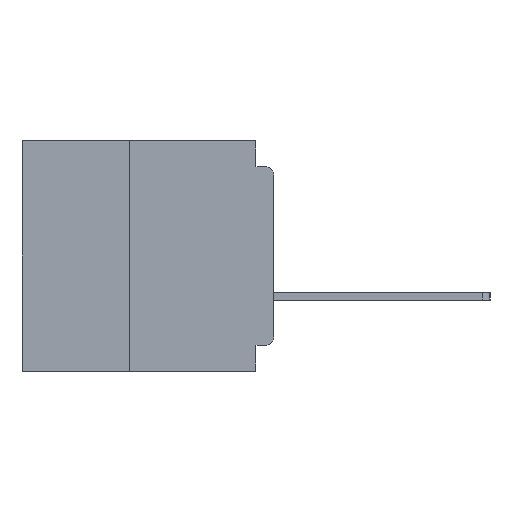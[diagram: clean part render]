
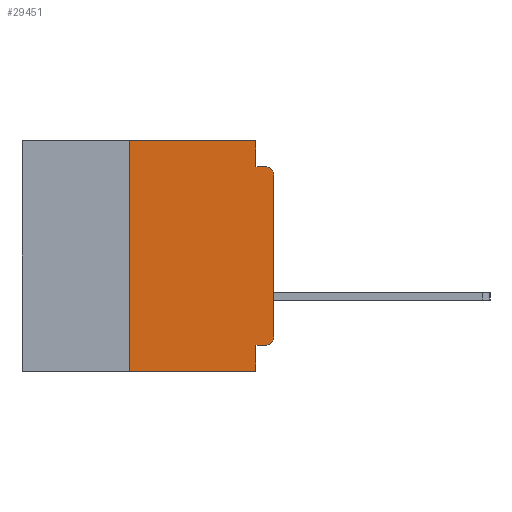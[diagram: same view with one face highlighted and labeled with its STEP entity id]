
A CAD part, left-side view. The second image highlights one B-rep face of the part: STEP entity #29451.
In plain terms, the highlighted planar face has unit normal (-1, 0, 0).
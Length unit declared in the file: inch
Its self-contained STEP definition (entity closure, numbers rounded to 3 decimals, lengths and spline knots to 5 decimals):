
#297 = VECTOR ( 'NONE', #43641, 39.37008 ) ;
#363 = DIRECTION ( 'NONE',  ( -1., 0., 0. ) ) ;
#499 = VERTEX_POINT ( 'NONE', #58375 ) ;
#901 = DIRECTION ( 'NONE',  ( 0., 0., -1. ) ) ;
#1110 = CARTESIAN_POINT ( 'NONE',  ( 0., 0.031, -0.4 ) ) ;
#2289 = CARTESIAN_POINT ( 'NONE',  ( 0., 0.031, -0.355 ) ) ;
#3205 = VERTEX_POINT ( 'NONE', #30571 ) ;
#4628 = EDGE_CURVE ( 'NONE', #499, #45607, #49005, .T. ) ;
#5086 = VECTOR ( 'NONE', #58828, 39.37008 ) ;
#6500 = EDGE_CURVE ( 'NONE', #499, #8777, #32813, .T. ) ;
#8254 = FACE_OUTER_BOUND ( 'NONE', #55263, .T. ) ;
#8302 = CARTESIAN_POINT ( 'NONE',  ( 0., 0., -0.34 ) ) ;
#8472 = CARTESIAN_POINT ( 'NONE',  ( 0., 0.031, -0.4 ) ) ;
#8777 = VERTEX_POINT ( 'NONE', #2289 ) ;
#8823 = VECTOR ( 'NONE', #19316, 39.37008 ) ;
#9510 = DIRECTION ( 'NONE',  ( 0., -1., 0. ) ) ;
#9801 = CARTESIAN_POINT ( 'NONE',  ( 0., 0., -0.045 ) ) ;
#10538 = ORIENTED_EDGE ( 'NONE', *, *, #6500, .F. ) ;
#11288 = ORIENTED_EDGE ( 'NONE', *, *, #31614, .T. ) ;
#12706 = ORIENTED_EDGE ( 'NONE', *, *, #37707, .F. ) ;
#13211 = VERTEX_POINT ( 'NONE', #19396 ) ;
#13712 = AXIS2_PLACEMENT_3D ( 'NONE', #56917, #27549, #61792 ) ;
#14845 = DIRECTION ( 'NONE',  ( 0., -1., 0. ) ) ;
#15233 = LINE ( 'NONE', #38761, #297 ) ;
#15885 = CARTESIAN_POINT ( 'NONE',  ( 0., 0.25, -0.4 ) ) ;
#19316 = DIRECTION ( 'NONE',  ( 0., 0., 1. ) ) ;
#19396 = CARTESIAN_POINT ( 'NONE',  ( 0., 0., -0.06 ) ) ;
#20513 = EDGE_CURVE ( 'NONE', #48472, #58981, #15233, .T. ) ;
#20899 = DIRECTION ( 'NONE',  ( 0., 0., 1. ) ) ;
#21132 = VECTOR ( 'NONE', #14845, 39.37008 ) ;
#23378 = CARTESIAN_POINT ( 'NONE',  ( 0., 0.031, 0. ) ) ;
#25372 = LINE ( 'NONE', #15885, #49978 ) ;
#26031 = VERTEX_POINT ( 'NONE', #8472 ) ;
#27549 = DIRECTION ( 'NONE',  ( -1., 0., 0. ) ) ;
#29451 = ADVANCED_FACE ( 'NONE', ( #8254 ), #57670, .F. ) ;
#29484 = CARTESIAN_POINT ( 'NONE',  ( 0., 0.437, -0.4 ) ) ;
#30360 = CARTESIAN_POINT ( 'NONE',  ( 0., 0.015, -0.34 ) ) ;
#30506 = ORIENTED_EDGE ( 'NONE', *, *, #43834, .T. ) ;
#30571 = CARTESIAN_POINT ( 'NONE',  ( 0., 0.25, 0. ) ) ;
#31138 = EDGE_CURVE ( 'NONE', #45115, #3205, #25372, .T. ) ;
#31614 = EDGE_CURVE ( 'NONE', #45607, #13211, #61322, .T. ) ;
#32395 = CARTESIAN_POINT ( 'NONE',  ( 0., 0.031, -0.045 ) ) ;
#32813 = LINE ( 'NONE', #50695, #58826 ) ;
#33079 = CARTESIAN_POINT ( 'NONE',  ( 0., 0.437, 0. ) ) ;
#33307 = DIRECTION ( 'NONE',  ( 0., 0., -1. ) ) ;
#34844 = LINE ( 'NONE', #29484, #5086 ) ;
#35324 = DIRECTION ( 'NONE',  ( 0., 0., -1. ) ) ;
#37707 = EDGE_CURVE ( 'NONE', #58981, #37766, #60367, .T. ) ;
#37766 = VERTEX_POINT ( 'NONE', #44688 ) ;
#38193 = ORIENTED_EDGE ( 'NONE', *, *, #51375, .T. ) ;
#38761 = CARTESIAN_POINT ( 'NONE',  ( 0., 0.031, 0. ) ) ;
#39537 = ORIENTED_EDGE ( 'NONE', *, *, #31138, .F. ) ;
#43641 = DIRECTION ( 'NONE',  ( 0., 0., -1. ) ) ;
#43834 = EDGE_CURVE ( 'NONE', #13211, #37766, #56960, .T. ) ;
#44688 = CARTESIAN_POINT ( 'NONE',  ( 0., 0.015, -0.045 ) ) ;
#45115 = VERTEX_POINT ( 'NONE', #58703 ) ;
#45207 = VECTOR ( 'NONE', #9510, 39.37008 ) ;
#45607 = VERTEX_POINT ( 'NONE', #8302 ) ;
#46761 = LINE ( 'NONE', #49159, #45207 ) ;
#47475 = AXIS2_PLACEMENT_3D ( 'NONE', #30360, #363, #35324 ) ;
#48472 = VERTEX_POINT ( 'NONE', #23378 ) ;
#48823 = ORIENTED_EDGE ( 'NONE', *, *, #4628, .T. ) ;
#48880 = LINE ( 'NONE', #1110, #61831 ) ;
#49005 = CIRCLE ( 'NONE', #47475, 0.015 ) ;
#49159 = CARTESIAN_POINT ( 'NONE',  ( 0., 0.437, 0. ) ) ;
#49428 = EDGE_CURVE ( 'NONE', #8777, #26031, #48880, .T. ) ;
#49978 = VECTOR ( 'NONE', #20899, 39.37008 ) ;
#50152 = AXIS2_PLACEMENT_3D ( 'NONE', #33079, #62545, #33307 ) ;
#50695 = CARTESIAN_POINT ( 'NONE',  ( 0., 0., -0.355 ) ) ;
#51375 = EDGE_CURVE ( 'NONE', #45115, #26031, #34844, .T. ) ;
#53790 = CARTESIAN_POINT ( 'NONE',  ( 0., 0., 0. ) ) ;
#54299 = EDGE_CURVE ( 'NONE', #3205, #48472, #46761, .T. ) ;
#55263 = EDGE_LOOP ( 'NONE', ( #11288, #30506, #12706, #61041, #61130, #39537, #38193, #57351, #10538, #48823 ) ) ;
#55634 = DIRECTION ( 'NONE',  ( 0., 1., 0. ) ) ;
#56917 = CARTESIAN_POINT ( 'NONE',  ( 0., 0.015, -0.06 ) ) ;
#56960 = CIRCLE ( 'NONE', #13712, 0.015 ) ;
#57351 = ORIENTED_EDGE ( 'NONE', *, *, #49428, .F. ) ;
#57670 = PLANE ( 'NONE',  #50152 ) ;
#58375 = CARTESIAN_POINT ( 'NONE',  ( 0., 0.015, -0.355 ) ) ;
#58703 = CARTESIAN_POINT ( 'NONE',  ( 0., 0.25, -0.4 ) ) ;
#58826 = VECTOR ( 'NONE', #55634, 39.37008 ) ;
#58828 = DIRECTION ( 'NONE',  ( 0., -1., 0. ) ) ;
#58981 = VERTEX_POINT ( 'NONE', #32395 ) ;
#60367 = LINE ( 'NONE', #9801, #21132 ) ;
#61041 = ORIENTED_EDGE ( 'NONE', *, *, #20513, .F. ) ;
#61130 = ORIENTED_EDGE ( 'NONE', *, *, #54299, .F. ) ;
#61322 = LINE ( 'NONE', #53790, #8823 ) ;
#61792 = DIRECTION ( 'NONE',  ( 0., 0., -1. ) ) ;
#61831 = VECTOR ( 'NONE', #901, 39.37008 ) ;
#62545 = DIRECTION ( 'NONE',  ( 1., 0., 0. ) ) ;
